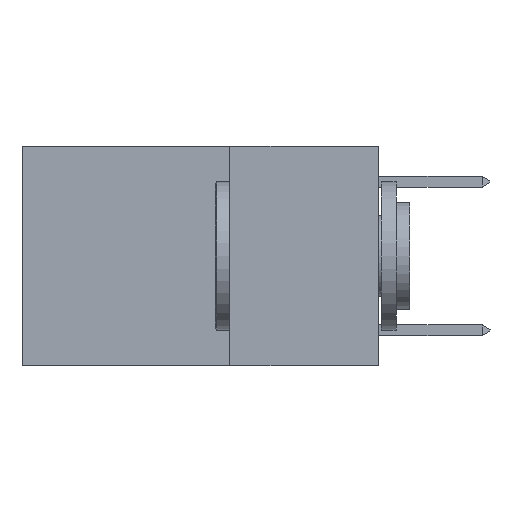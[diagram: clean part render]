
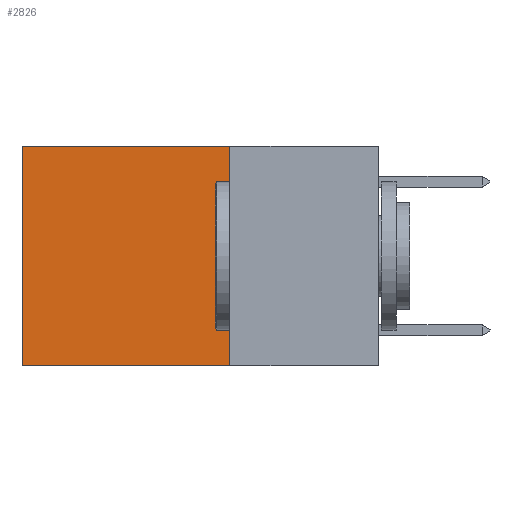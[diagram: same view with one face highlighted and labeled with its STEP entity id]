
A CAD part, left-side view. The second image highlights one B-rep face of the part: STEP entity #2826.
In plain terms, the highlighted planar face has unit normal (-1, 0, 0).
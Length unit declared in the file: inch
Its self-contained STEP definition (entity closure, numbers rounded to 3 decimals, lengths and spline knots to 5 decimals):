
#910 = CARTESIAN_POINT ( 'NONE',  ( 0.2625, 0.25, 0. ) ) ;
#1852 = CARTESIAN_POINT ( 'NONE',  ( 0.2625, 0.25, 0. ) ) ;
#1883 = PLANE ( 'NONE',  #23867 ) ;
#1985 = ORIENTED_EDGE ( 'NONE', *, *, #21420, .F. ) ;
#2174 = DIRECTION ( 'NONE',  ( 0., 0., -1. ) ) ;
#2826 = ADVANCED_FACE ( 'NONE', ( #18626 ), #1883, .F. ) ;
#3506 = ORIENTED_EDGE ( 'NONE', *, *, #7554, .T. ) ;
#5454 = VERTEX_POINT ( 'NONE', #13085 ) ;
#6240 = EDGE_CURVE ( 'NONE', #8765, #15166, #18445, .T. ) ;
#6689 = CARTESIAN_POINT ( 'NONE',  ( 0.2625, 0.6, 0. ) ) ;
#7312 = DIRECTION ( 'NONE',  ( 0., 1., 0. ) ) ;
#7457 = DIRECTION ( 'NONE',  ( 0., 1., 0. ) ) ;
#7554 = EDGE_CURVE ( 'NONE', #5454, #15166, #19730, .T. ) ;
#8765 = VERTEX_POINT ( 'NONE', #23930 ) ;
#9368 = CARTESIAN_POINT ( 'NONE',  ( 0.2625, 0.25, -0.37 ) ) ;
#10411 = CARTESIAN_POINT ( 'NONE',  ( 0.2625, 0.25, 0. ) ) ;
#12759 = CARTESIAN_POINT ( 'NONE',  ( 0.2625, 0.6, -0.37 ) ) ;
#12767 = VECTOR ( 'NONE', #7312, 39.37008 ) ;
#13085 = CARTESIAN_POINT ( 'NONE',  ( 0.2625, 0.6, 0. ) ) ;
#15115 = DIRECTION ( 'NONE',  ( 0., 0., -1. ) ) ;
#15166 = VERTEX_POINT ( 'NONE', #12759 ) ;
#18357 = LINE ( 'NONE', #24085, #27009 ) ;
#18445 = LINE ( 'NONE', #9368, #12767 ) ;
#18544 = ORIENTED_EDGE ( 'NONE', *, *, #21792, .T. ) ;
#18626 = FACE_OUTER_BOUND ( 'NONE', #26200, .T. ) ;
#18984 = ORIENTED_EDGE ( 'NONE', *, *, #6240, .F. ) ;
#19730 = LINE ( 'NONE', #6689, #25039 ) ;
#21344 = DIRECTION ( 'NONE',  ( 1., 0., 0. ) ) ;
#21420 = EDGE_CURVE ( 'NONE', #24740, #8765, #22375, .T. ) ;
#21792 = EDGE_CURVE ( 'NONE', #24740, #5454, #18357, .T. ) ;
#22030 = VECTOR ( 'NONE', #15115, 39.37008 ) ;
#22375 = LINE ( 'NONE', #1852, #22030 ) ;
#23785 = DIRECTION ( 'NONE',  ( 0., 0., -1. ) ) ;
#23867 = AXIS2_PLACEMENT_3D ( 'NONE', #10411, #21344, #2174 ) ;
#23930 = CARTESIAN_POINT ( 'NONE',  ( 0.2625, 0.25, -0.37 ) ) ;
#24085 = CARTESIAN_POINT ( 'NONE',  ( 0.2625, 0.25, 0. ) ) ;
#24740 = VERTEX_POINT ( 'NONE', #910 ) ;
#25039 = VECTOR ( 'NONE', #23785, 39.37008 ) ;
#26200 = EDGE_LOOP ( 'NONE', ( #3506, #18984, #1985, #18544 ) ) ;
#27009 = VECTOR ( 'NONE', #7457, 39.37008 ) ;
